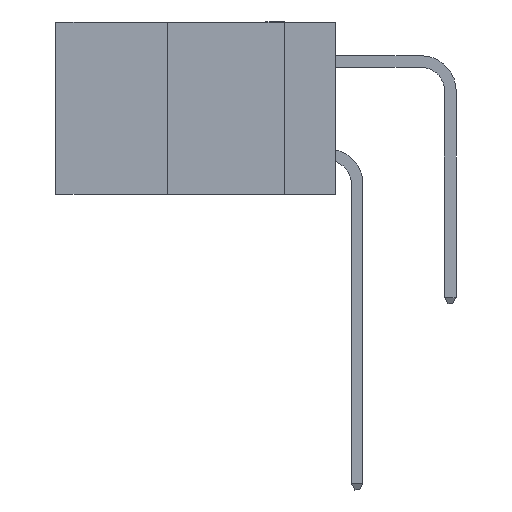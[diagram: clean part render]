
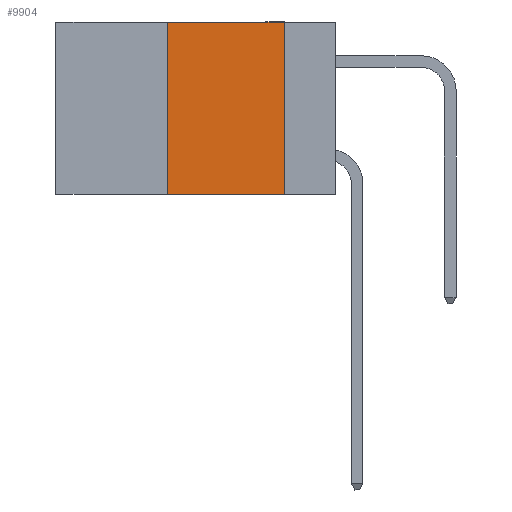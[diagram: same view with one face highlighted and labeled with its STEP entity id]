
A CAD part, left-side view. The second image highlights one B-rep face of the part: STEP entity #9904.
In plain terms, the highlighted planar face has unit normal (-1, 0, 0).
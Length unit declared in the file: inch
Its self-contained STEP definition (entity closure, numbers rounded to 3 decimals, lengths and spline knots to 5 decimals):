
#663 = VERTEX_POINT ( 'NONE', #6403 ) ;
#1208 = DIRECTION ( 'NONE',  ( 1., 0., 0. ) ) ;
#1322 = PLANE ( 'NONE',  #14563 ) ;
#1348 = DIRECTION ( 'NONE',  ( 0., 0., 1. ) ) ;
#1953 = VERTEX_POINT ( 'NONE', #2323 ) ;
#2323 = CARTESIAN_POINT ( 'NONE',  ( 0., 0.36, -0.37 ) ) ;
#2549 = CARTESIAN_POINT ( 'NONE',  ( 0., 0.6, 0. ) ) ;
#3312 = VECTOR ( 'NONE', #9655, 39.37008 ) ;
#3899 = DIRECTION ( 'NONE',  ( 0., 0., -1. ) ) ;
#4970 = EDGE_LOOP ( 'NONE', ( #14843, #8164, #11101, #9484 ) ) ;
#6286 = VERTEX_POINT ( 'NONE', #14566 ) ;
#6403 = CARTESIAN_POINT ( 'NONE',  ( 0., 0.36, 0. ) ) ;
#8164 = ORIENTED_EDGE ( 'NONE', *, *, #13553, .F. ) ;
#8271 = LINE ( 'NONE', #12297, #14512 ) ;
#8321 = FACE_OUTER_BOUND ( 'NONE', #4970, .T. ) ;
#8423 = VECTOR ( 'NONE', #8746, 39.37008 ) ;
#8746 = DIRECTION ( 'NONE',  ( 0., -1., 0. ) ) ;
#8808 = LINE ( 'NONE', #11320, #8423 ) ;
#8987 = EDGE_CURVE ( 'NONE', #1953, #663, #16537, .T. ) ;
#9484 = ORIENTED_EDGE ( 'NONE', *, *, #11987, .T. ) ;
#9655 = DIRECTION ( 'NONE',  ( 0., -1., 0. ) ) ;
#9904 = ADVANCED_FACE ( 'NONE', ( #8321 ), #1322, .F. ) ;
#10942 = EDGE_CURVE ( 'NONE', #6286, #12952, #8271, .T. ) ;
#11101 = ORIENTED_EDGE ( 'NONE', *, *, #8987, .F. ) ;
#11320 = CARTESIAN_POINT ( 'NONE',  ( 0., 0.6, 0. ) ) ;
#11685 = CARTESIAN_POINT ( 'NONE',  ( 0., 0.6, -0.37 ) ) ;
#11735 = VECTOR ( 'NONE', #1348, 39.37008 ) ;
#11853 = LINE ( 'NONE', #11685, #3312 ) ;
#11987 = EDGE_CURVE ( 'NONE', #1953, #12952, #11853, .T. ) ;
#12017 = CARTESIAN_POINT ( 'NONE',  ( 0., 0.11, -0.37 ) ) ;
#12297 = CARTESIAN_POINT ( 'NONE',  ( 0., 0.11, 0. ) ) ;
#12952 = VERTEX_POINT ( 'NONE', #12017 ) ;
#13553 = EDGE_CURVE ( 'NONE', #663, #6286, #8808, .T. ) ;
#14512 = VECTOR ( 'NONE', #14796, 39.37008 ) ;
#14517 = CARTESIAN_POINT ( 'NONE',  ( 0., 0.36, 0. ) ) ;
#14563 = AXIS2_PLACEMENT_3D ( 'NONE', #2549, #1208, #3899 ) ;
#14566 = CARTESIAN_POINT ( 'NONE',  ( 0., 0.11, 0. ) ) ;
#14796 = DIRECTION ( 'NONE',  ( 0., 0., -1. ) ) ;
#14843 = ORIENTED_EDGE ( 'NONE', *, *, #10942, .F. ) ;
#16537 = LINE ( 'NONE', #14517, #11735 ) ;
